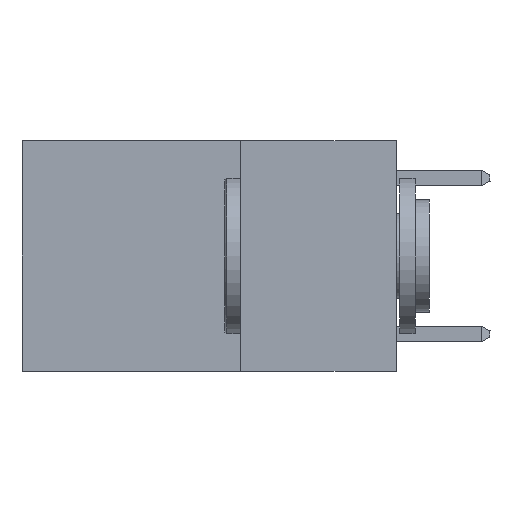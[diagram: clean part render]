
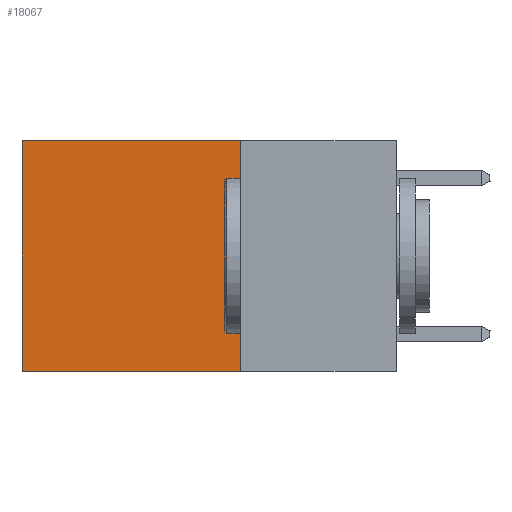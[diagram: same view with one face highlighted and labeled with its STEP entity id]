
A CAD part, left-side view. The second image highlights one B-rep face of the part: STEP entity #18067.
In plain terms, the highlighted planar face has unit normal (-1, 0, 0).
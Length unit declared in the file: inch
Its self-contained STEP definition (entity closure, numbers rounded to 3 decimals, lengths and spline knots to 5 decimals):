
#601 = VECTOR ( 'NONE', #15260, 39.37008 ) ;
#743 = CARTESIAN_POINT ( 'NONE',  ( 0.2625, 0.6, -0.37 ) ) ;
#990 = VECTOR ( 'NONE', #5192, 39.37008 ) ;
#2120 = CARTESIAN_POINT ( 'NONE',  ( 0.2625, 0.25, 0. ) ) ;
#2194 = EDGE_CURVE ( 'NONE', #11773, #12675, #4194, .T. ) ;
#2665 = LINE ( 'NONE', #10865, #7263 ) ;
#3085 = PLANE ( 'NONE',  #14249 ) ;
#3541 = CARTESIAN_POINT ( 'NONE',  ( 0.2625, 0.6, 0. ) ) ;
#3564 = VERTEX_POINT ( 'NONE', #2120 ) ;
#3716 = FACE_OUTER_BOUND ( 'NONE', #16275, .T. ) ;
#4194 = LINE ( 'NONE', #10252, #11177 ) ;
#4434 = EDGE_CURVE ( 'NONE', #3564, #19629, #2665, .T. ) ;
#4822 = EDGE_CURVE ( 'NONE', #19629, #12675, #15278, .T. ) ;
#5192 = DIRECTION ( 'NONE',  ( 0., 0., -1. ) ) ;
#7263 = VECTOR ( 'NONE', #19958, 39.37008 ) ;
#8434 = EDGE_CURVE ( 'NONE', #3564, #11773, #13104, .T. ) ;
#10252 = CARTESIAN_POINT ( 'NONE',  ( 0.2625, 0.25, -0.37 ) ) ;
#10865 = CARTESIAN_POINT ( 'NONE',  ( 0.2625, 0.25, 0. ) ) ;
#11177 = VECTOR ( 'NONE', #18291, 39.37008 ) ;
#11773 = VERTEX_POINT ( 'NONE', #21124 ) ;
#12675 = VERTEX_POINT ( 'NONE', #743 ) ;
#12812 = DIRECTION ( 'NONE',  ( 1., 0., 0. ) ) ;
#13104 = LINE ( 'NONE', #16815, #990 ) ;
#14249 = AXIS2_PLACEMENT_3D ( 'NONE', #21084, #12812, #19463 ) ;
#14416 = CARTESIAN_POINT ( 'NONE',  ( 0.2625, 0.6, 0. ) ) ;
#15260 = DIRECTION ( 'NONE',  ( 0., 0., -1. ) ) ;
#15278 = LINE ( 'NONE', #14416, #601 ) ;
#16275 = EDGE_LOOP ( 'NONE', ( #18768, #18285, #17694, #20306 ) ) ;
#16815 = CARTESIAN_POINT ( 'NONE',  ( 0.2625, 0.25, 0. ) ) ;
#17694 = ORIENTED_EDGE ( 'NONE', *, *, #8434, .F. ) ;
#18067 = ADVANCED_FACE ( 'NONE', ( #3716 ), #3085, .F. ) ;
#18285 = ORIENTED_EDGE ( 'NONE', *, *, #2194, .F. ) ;
#18291 = DIRECTION ( 'NONE',  ( 0., 1., 0. ) ) ;
#18768 = ORIENTED_EDGE ( 'NONE', *, *, #4822, .T. ) ;
#19463 = DIRECTION ( 'NONE',  ( 0., 0., -1. ) ) ;
#19629 = VERTEX_POINT ( 'NONE', #3541 ) ;
#19958 = DIRECTION ( 'NONE',  ( 0., 1., 0. ) ) ;
#20306 = ORIENTED_EDGE ( 'NONE', *, *, #4434, .T. ) ;
#21084 = CARTESIAN_POINT ( 'NONE',  ( 0.2625, 0.25, 0. ) ) ;
#21124 = CARTESIAN_POINT ( 'NONE',  ( 0.2625, 0.25, -0.37 ) ) ;
